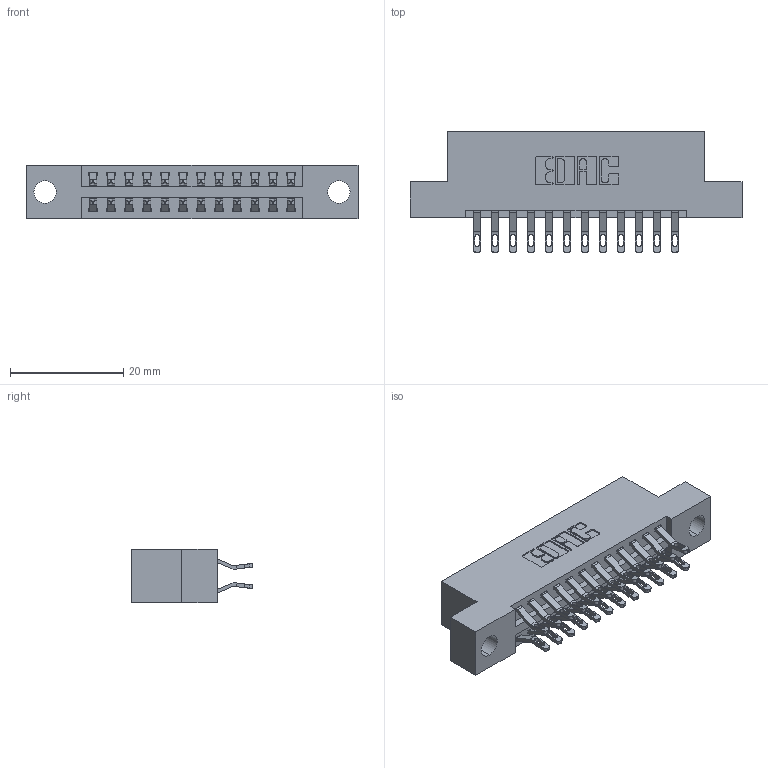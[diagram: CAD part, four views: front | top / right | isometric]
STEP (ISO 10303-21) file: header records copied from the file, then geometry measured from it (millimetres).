
FILE_DESCRIPTION (( 'STEP AP203' ), '1' );
FILE_NAME ('346-024-555-204.STEP', '2022-05-18T23:52:08', ( '' ), ( '' ), 'SwSTEP 2.0', 'SolidWorks 2020', '' );
FILE_SCHEMA (( 'CONFIG_CONTROL_DESIGN' ));
Length unit declared in the file: inch
Products named in the file (3): 345-292-001_555 Tail; 346 Part_Flush Mounting Lugs - 0.156 Dia-TH; 346-024-555-204
Assembly tree (25 placements, depth 2):
  346-024-555-204
    346 Part_Flush Mounting Lugs - 0.156 Dia-TH
    345-292-001_555 Tail  x24
Bounding box: 58.67 x 21.46 x 9.4 mm (x, y, z)
Volume: 5452.1 mm3; surface area: 7118.8 mm2
Topology: 25 solids, 25 shells, 1528 faces, 4757 edges, 3170 vertices
Faces by surface type: plane 882, cylinder 646
Entity records: 12615 total; most frequent: CARTESIAN_POINT 2160, ORIENTED_EDGE 2062, DIRECTION 1923, EDGE_CURVE 1031, VECTOR 831, LINE 831, VERTEX_POINT 686, AXIS2_PLACEMENT_3D 546
